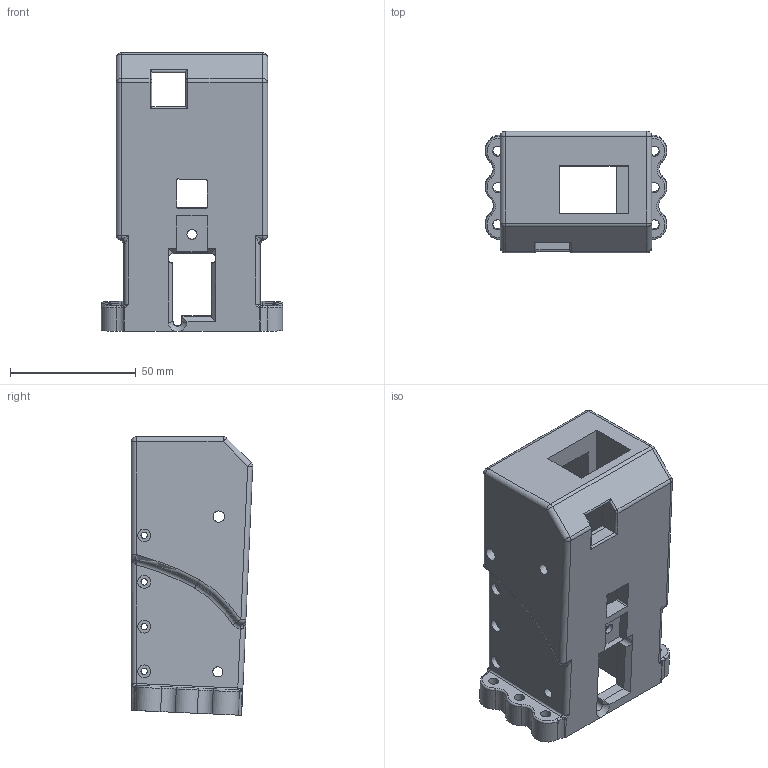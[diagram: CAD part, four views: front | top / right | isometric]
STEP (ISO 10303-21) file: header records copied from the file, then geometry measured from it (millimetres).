
FILE_DESCRIPTION(/* description */ (''),/* implementation_level */ '2;1');
FILE_NAME(/* name */ 'Plastikov v0.9 Rear Receiver.stp',/* time_stamp */ '2019-12-22T15:33:43-06:00',/* author */ ('johne'),/* organization */ (''),/* preprocessor_version */ 'ST-DEVELOPER v18',/* originating_system */ 'Autodesk Inventor 2020',/* authorisation */ '');
FILE_SCHEMA (('AUTOMOTIVE_DESIGN { 1 0 10303 214 3 1 1 }'));
Length unit declared in the file: millimetre
Products named in the file (1): Rear half alt
Bounding box: 72.2 x 48.28 x 110.76 mm (x, y, z)
Volume: 147684.5 mm3; surface area: 38813.1 mm2
Topology: 1 solids, 1 shells, 222 faces, 585 edges, 365 vertices
Faces by surface type: cylinder 85, plane 69, torus 27, bspline 26, sphere 14, cone 1
Full cylindrical faces by diameter (mm): 2.5 x8, 3.12 x4, 4 x9, 4.5 x2, 5.08 x8
Entity records: 7637 total; most frequent: CARTESIAN_POINT 1978, DIRECTION 1210, ORIENTED_EDGE 1154, EDGE_CURVE 577, AXIS2_PLACEMENT_3D 481, VERTEX_POINT 365, EDGE_LOOP 276, CIRCLE 262
